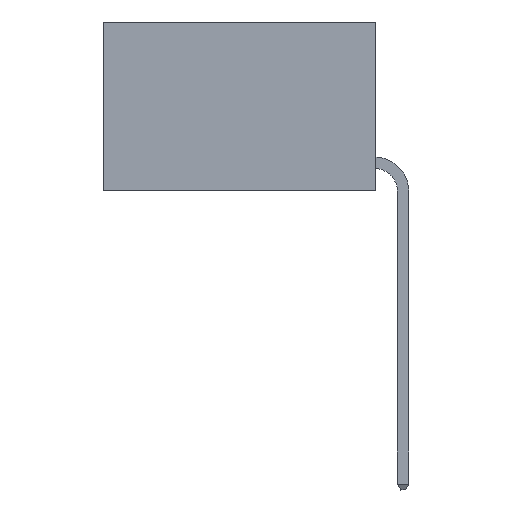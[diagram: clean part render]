
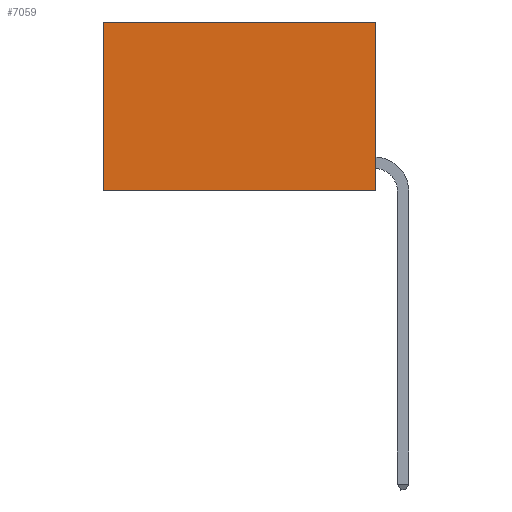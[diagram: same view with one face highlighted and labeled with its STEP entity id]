
A CAD part, left-side view. The second image highlights one B-rep face of the part: STEP entity #7059.
In plain terms, the highlighted planar face has unit normal (-1, 0, 0).
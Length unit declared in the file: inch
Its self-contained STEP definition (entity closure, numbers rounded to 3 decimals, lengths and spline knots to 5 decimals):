
#338 = EDGE_CURVE ( 'NONE', #983, #7925, #6954, .T. ) ;
#689 = VERTEX_POINT ( 'NONE', #757 ) ;
#757 = CARTESIAN_POINT ( 'NONE',  ( 0.2625, 0.6, 0. ) ) ;
#983 = VERTEX_POINT ( 'NONE', #7389 ) ;
#2014 = DIRECTION ( 'NONE',  ( 1., 0., 0. ) ) ;
#2063 = DIRECTION ( 'NONE',  ( 0., 0., -1. ) ) ;
#2178 = DIRECTION ( 'NONE',  ( 0., 0., -1. ) ) ;
#2289 = LINE ( 'NONE', #9736, #4209 ) ;
#3171 = DIRECTION ( 'NONE',  ( 0., 1., 0. ) ) ;
#3616 = LINE ( 'NONE', #6981, #10145 ) ;
#3838 = DIRECTION ( 'NONE',  ( 0., 0., -1. ) ) ;
#3900 = VERTEX_POINT ( 'NONE', #4046 ) ;
#3954 = EDGE_CURVE ( 'NONE', #689, #7925, #2289, .T. ) ;
#3984 = LINE ( 'NONE', #6474, #7728 ) ;
#4046 = CARTESIAN_POINT ( 'NONE',  ( 0.2625, 0., 0. ) ) ;
#4209 = VECTOR ( 'NONE', #3838, 39.37008 ) ;
#4693 = FACE_OUTER_BOUND ( 'NONE', #8424, .T. ) ;
#4749 = DIRECTION ( 'NONE',  ( 0., 1., 0. ) ) ;
#5226 = ORIENTED_EDGE ( 'NONE', *, *, #3954, .T. ) ;
#5335 = ORIENTED_EDGE ( 'NONE', *, *, #7182, .T. ) ;
#6188 = PLANE ( 'NONE',  #8260 ) ;
#6474 = CARTESIAN_POINT ( 'NONE',  ( 0.2625, 0., 0. ) ) ;
#6954 = LINE ( 'NONE', #10742, #8220 ) ;
#6981 = CARTESIAN_POINT ( 'NONE',  ( 0.2625, 0., 0. ) ) ;
#7059 = ADVANCED_FACE ( 'NONE', ( #4693 ), #6188, .F. ) ;
#7182 = EDGE_CURVE ( 'NONE', #3900, #689, #3984, .T. ) ;
#7389 = CARTESIAN_POINT ( 'NONE',  ( 0.2625, 0., -0.37 ) ) ;
#7728 = VECTOR ( 'NONE', #3171, 39.37008 ) ;
#7925 = VERTEX_POINT ( 'NONE', #8980 ) ;
#8220 = VECTOR ( 'NONE', #4749, 39.37008 ) ;
#8260 = AXIS2_PLACEMENT_3D ( 'NONE', #9566, #2014, #2063 ) ;
#8424 = EDGE_LOOP ( 'NONE', ( #5226, #8627, #8687, #5335 ) ) ;
#8627 = ORIENTED_EDGE ( 'NONE', *, *, #338, .F. ) ;
#8687 = ORIENTED_EDGE ( 'NONE', *, *, #9424, .F. ) ;
#8980 = CARTESIAN_POINT ( 'NONE',  ( 0.2625, 0.6, -0.37 ) ) ;
#9424 = EDGE_CURVE ( 'NONE', #3900, #983, #3616, .T. ) ;
#9566 = CARTESIAN_POINT ( 'NONE',  ( 0.2625, 0., 0. ) ) ;
#9736 = CARTESIAN_POINT ( 'NONE',  ( 0.2625, 0.6, 0. ) ) ;
#10145 = VECTOR ( 'NONE', #2178, 39.37008 ) ;
#10742 = CARTESIAN_POINT ( 'NONE',  ( 0.2625, 0., -0.37 ) ) ;
